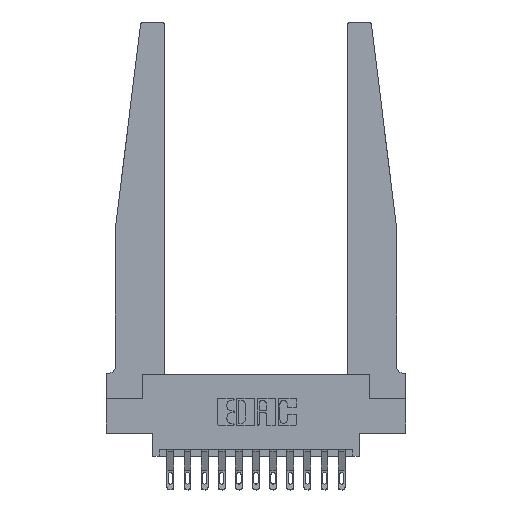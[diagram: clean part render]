
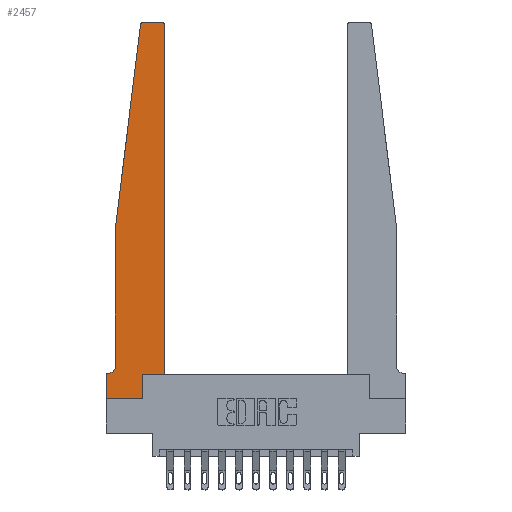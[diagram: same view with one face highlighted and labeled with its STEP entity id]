
A CAD part, top view. The second image highlights one B-rep face of the part: STEP entity #2457.
In plain terms, the highlighted planar face has unit normal (0, 0, 1).
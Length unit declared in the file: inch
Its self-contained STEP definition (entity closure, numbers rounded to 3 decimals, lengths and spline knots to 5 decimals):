
#323 = ORIENTED_EDGE ( 'NONE', *, *, #1003, .T. ) ;
#482 = PLANE ( 'NONE',  #2604 ) ;
#499 = DIRECTION ( 'NONE',  ( -1., 0., 0. ) ) ;
#708 = ORIENTED_EDGE ( 'NONE', *, *, #10986, .T. ) ;
#981 = CARTESIAN_POINT ( 'NONE',  ( 0.2605, 0.18, 0.37 ) ) ;
#1003 = EDGE_CURVE ( 'NONE', #10655, #13580, #6608, .T. ) ;
#1150 = EDGE_CURVE ( 'NONE', #3509, #9303, #12040, .T. ) ;
#1327 = DIRECTION ( 'NONE',  ( -1., 0., 0. ) ) ;
#1751 = VECTOR ( 'NONE', #499, 39.37008 ) ;
#1808 = ORIENTED_EDGE ( 'NONE', *, *, #1150, .T. ) ;
#1917 = CARTESIAN_POINT ( 'NONE',  ( 0.2605, 0.18, 0.37 ) ) ;
#2040 = VERTEX_POINT ( 'NONE', #981 ) ;
#2295 = DIRECTION ( 'NONE',  ( 0., -1., 0. ) ) ;
#2346 = CARTESIAN_POINT ( 'NONE',  ( 0., 0., 0.37 ) ) ;
#2457 = ADVANCED_FACE ( 'NONE', ( #12298 ), #482, .T. ) ;
#2522 = EDGE_CURVE ( 'NONE', #10496, #13853, #14712, .T. ) ;
#2604 = AXIS2_PLACEMENT_3D ( 'NONE', #13748, #3178, #3018 ) ;
#2646 = DIRECTION ( 'NONE',  ( 0., 0., -1. ) ) ;
#3018 = DIRECTION ( 'NONE',  ( 1., 0., 0. ) ) ;
#3178 = DIRECTION ( 'NONE',  ( 0., 0., 1. ) ) ;
#3354 = DIRECTION ( 'NONE',  ( 1., 0., 0. ) ) ;
#3477 = CARTESIAN_POINT ( 'NONE',  ( 0.395, 2.72, 0.37 ) ) ;
#3509 = VERTEX_POINT ( 'NONE', #10668 ) ;
#3943 = CARTESIAN_POINT ( 'NONE',  ( 0.425, 0.18, 0.37 ) ) ;
#4254 = LINE ( 'NONE', #10639, #16319 ) ;
#4646 = AXIS2_PLACEMENT_3D ( 'NONE', #3477, #12668, #14234 ) ;
#4725 = VECTOR ( 'NONE', #10870, 39.37008 ) ;
#4832 = AXIS2_PLACEMENT_3D ( 'NONE', #15054, #6771, #5514 ) ;
#4858 = EDGE_CURVE ( 'NONE', #8625, #3509, #6762, .T. ) ;
#4991 = CARTESIAN_POINT ( 'NONE',  ( 0.065, 1.25, 0.37 ) ) ;
#5399 = CARTESIAN_POINT ( 'NONE',  ( 0., 0., 0.37 ) ) ;
#5514 = DIRECTION ( 'NONE',  ( 1., 0., 0. ) ) ;
#5918 = CARTESIAN_POINT ( 'NONE',  ( 0., 0., 0.37 ) ) ;
#6219 = LINE ( 'NONE', #2346, #8653 ) ;
#6608 = LINE ( 'NONE', #15770, #12897 ) ;
#6762 = LINE ( 'NONE', #3943, #13084 ) ;
#6771 = DIRECTION ( 'NONE',  ( 0., 0., 1. ) ) ;
#7141 = CARTESIAN_POINT ( 'NONE',  ( 0.395, 2.75, 0.37 ) ) ;
#7958 = LINE ( 'NONE', #5399, #4725 ) ;
#8027 = ORIENTED_EDGE ( 'NONE', *, *, #10959, .T. ) ;
#8069 = AXIS2_PLACEMENT_3D ( 'NONE', #10472, #2646, #1327 ) ;
#8084 = DIRECTION ( 'NONE',  ( -1., 0., 0. ) ) ;
#8207 = LINE ( 'NONE', #13383, #15176 ) ;
#8493 = CARTESIAN_POINT ( 'NONE',  ( 0.425, 0.18, 0.37 ) ) ;
#8612 = CARTESIAN_POINT ( 'NONE',  ( 0.25, 2.75, 0.37 ) ) ;
#8625 = VERTEX_POINT ( 'NONE', #8493 ) ;
#8653 = VECTOR ( 'NONE', #16908, 39.37008 ) ;
#8864 = LINE ( 'NONE', #4991, #14060 ) ;
#9179 = VERTEX_POINT ( 'NONE', #15517 ) ;
#9197 = CARTESIAN_POINT ( 'NONE',  ( 0.015, 0.1875, 0.37 ) ) ;
#9205 = CARTESIAN_POINT ( 'NONE',  ( 0.065, 0.2375, 0.37 ) ) ;
#9275 = LINE ( 'NONE', #1917, #14444 ) ;
#9303 = VERTEX_POINT ( 'NONE', #7141 ) ;
#9374 = CARTESIAN_POINT ( 'NONE',  ( 0.27653, 2.75, 0.37 ) ) ;
#9627 = EDGE_CURVE ( 'NONE', #12237, #2040, #9275, .T. ) ;
#9741 = LINE ( 'NONE', #8612, #1751 ) ;
#10299 = DIRECTION ( 'NONE',  ( 0., 1., 0. ) ) ;
#10374 = ORIENTED_EDGE ( 'NONE', *, *, #14171, .T. ) ;
#10471 = ORIENTED_EDGE ( 'NONE', *, *, #13607, .T. ) ;
#10472 = CARTESIAN_POINT ( 'NONE',  ( 0.015, 0.2375, 0.37 ) ) ;
#10496 = VERTEX_POINT ( 'NONE', #9374 ) ;
#10639 = CARTESIAN_POINT ( 'NONE',  ( 0.065, 1.25, 0.37 ) ) ;
#10655 = VERTEX_POINT ( 'NONE', #9197 ) ;
#10668 = CARTESIAN_POINT ( 'NONE',  ( 0.425, 2.72, 0.37 ) ) ;
#10870 = DIRECTION ( 'NONE',  ( 1., 0., 0. ) ) ;
#10959 = EDGE_CURVE ( 'NONE', #12342, #12237, #7958, .T. ) ;
#10986 = EDGE_CURVE ( 'NONE', #9179, #12418, #8864, .T. ) ;
#11066 = ORIENTED_EDGE ( 'NONE', *, *, #9627, .T. ) ;
#11257 = EDGE_CURVE ( 'NONE', #2040, #8625, #8207, .T. ) ;
#11444 = CARTESIAN_POINT ( 'NONE',  ( 0.2605, 0., 0.37 ) ) ;
#11875 = ORIENTED_EDGE ( 'NONE', *, *, #2522, .T. ) ;
#11959 = EDGE_LOOP ( 'NONE', ( #10471, #11875, #16684, #708, #15232, #323, #10374, #8027, #11066, #13834, #14099, #1808 ) ) ;
#12040 = CIRCLE ( 'NONE', #4646, 0.03 ) ;
#12184 = CIRCLE ( 'NONE', #8069, 0.05 ) ;
#12237 = VERTEX_POINT ( 'NONE', #11444 ) ;
#12298 = FACE_OUTER_BOUND ( 'NONE', #11959, .T. ) ;
#12342 = VERTEX_POINT ( 'NONE', #5918 ) ;
#12418 = VERTEX_POINT ( 'NONE', #9205 ) ;
#12668 = DIRECTION ( 'NONE',  ( 0., 0., 1. ) ) ;
#12897 = VECTOR ( 'NONE', #8084, 39.37008 ) ;
#13084 = VECTOR ( 'NONE', #10299, 39.37008 ) ;
#13254 = EDGE_CURVE ( 'NONE', #12418, #10655, #12184, .T. ) ;
#13275 = EDGE_CURVE ( 'NONE', #13853, #9179, #4254, .T. ) ;
#13383 = CARTESIAN_POINT ( 'NONE',  ( 0.425, 0.18, 0.37 ) ) ;
#13580 = VERTEX_POINT ( 'NONE', #15962 ) ;
#13607 = EDGE_CURVE ( 'NONE', #9303, #10496, #9741, .T. ) ;
#13748 = CARTESIAN_POINT ( 'NONE',  ( 0., 0.1875, 0.37 ) ) ;
#13834 = ORIENTED_EDGE ( 'NONE', *, *, #11257, .T. ) ;
#13853 = VERTEX_POINT ( 'NONE', #14426 ) ;
#14060 = VECTOR ( 'NONE', #2295, 39.37008 ) ;
#14099 = ORIENTED_EDGE ( 'NONE', *, *, #4858, .T. ) ;
#14171 = EDGE_CURVE ( 'NONE', #13580, #12342, #6219, .T. ) ;
#14234 = DIRECTION ( 'NONE',  ( 1., 0., 0. ) ) ;
#14426 = CARTESIAN_POINT ( 'NONE',  ( 0.24675, 2.72367, 0.37 ) ) ;
#14444 = VECTOR ( 'NONE', #16385, 39.37008 ) ;
#14712 = CIRCLE ( 'NONE', #4832, 0.03 ) ;
#15054 = CARTESIAN_POINT ( 'NONE',  ( 0.27653, 2.72, 0.37 ) ) ;
#15176 = VECTOR ( 'NONE', #3354, 39.37008 ) ;
#15232 = ORIENTED_EDGE ( 'NONE', *, *, #13254, .T. ) ;
#15517 = CARTESIAN_POINT ( 'NONE',  ( 0.065, 1.25, 0.37 ) ) ;
#15770 = CARTESIAN_POINT ( 'NONE',  ( 0.065, 0.1875, 0.37 ) ) ;
#15910 = DIRECTION ( 'NONE',  ( -0.122, -0.992, 0. ) ) ;
#15962 = CARTESIAN_POINT ( 'NONE',  ( 0., 0.1875, 0.37 ) ) ;
#16319 = VECTOR ( 'NONE', #15910, 39.37008 ) ;
#16385 = DIRECTION ( 'NONE',  ( 0., 1., 0. ) ) ;
#16684 = ORIENTED_EDGE ( 'NONE', *, *, #13275, .T. ) ;
#16908 = DIRECTION ( 'NONE',  ( 0., -1., 0. ) ) ;
